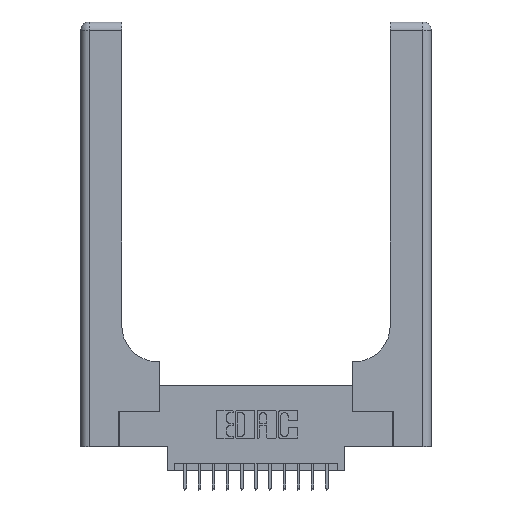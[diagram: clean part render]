
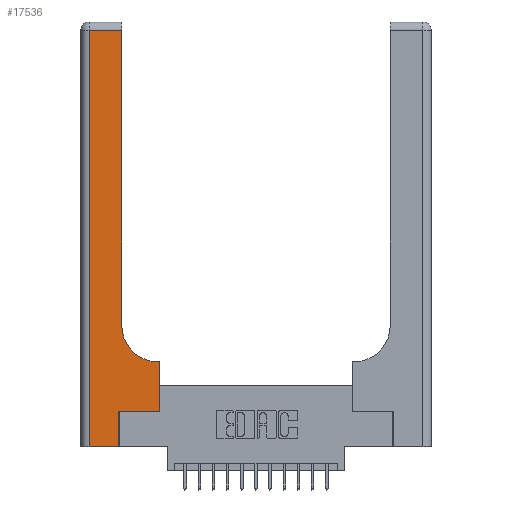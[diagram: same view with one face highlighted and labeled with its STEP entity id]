
A CAD part, top view. The second image highlights one B-rep face of the part: STEP entity #17536.
In plain terms, the highlighted planar face has unit normal (0, 0, 1).
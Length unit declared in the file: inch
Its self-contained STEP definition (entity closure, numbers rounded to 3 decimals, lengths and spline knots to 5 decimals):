
#185 = CIRCLE ( 'NONE', #14574, 0.25 ) ;
#428 = VERTEX_POINT ( 'NONE', #13243 ) ;
#440 = DIRECTION ( 'NONE',  ( 1., 0., 0. ) ) ;
#572 = LINE ( 'NONE', #4904, #17572 ) ;
#699 = EDGE_LOOP ( 'NONE', ( #13383, #5843, #14228, #2936, #4635, #8428, #7932, #6070, #11834 ) ) ;
#736 = LINE ( 'NONE', #6343, #16809 ) ;
#1186 = CARTESIAN_POINT ( 'NONE',  ( 0., 0., 0.37 ) ) ;
#1475 = EDGE_CURVE ( 'NONE', #5030, #13446, #18220, .T. ) ;
#1550 = VECTOR ( 'NONE', #15448, 39.37008 ) ;
#1582 = LINE ( 'NONE', #9690, #9158 ) ;
#1612 = DIRECTION ( 'NONE',  ( 0., -1., 0. ) ) ;
#1633 = VECTOR ( 'NONE', #12457, 39.37008 ) ;
#1812 = CARTESIAN_POINT ( 'NONE',  ( 0.5415, 0.85, 0.37 ) ) ;
#2524 = CARTESIAN_POINT ( 'NONE',  ( 0.269, 0.25, 0.37 ) ) ;
#2936 = ORIENTED_EDGE ( 'NONE', *, *, #12103, .T. ) ;
#4201 = LINE ( 'NONE', #1186, #4261 ) ;
#4261 = VECTOR ( 'NONE', #9842, 39.37008 ) ;
#4392 = VERTEX_POINT ( 'NONE', #14958 ) ;
#4635 = ORIENTED_EDGE ( 'NONE', *, *, #18204, .T. ) ;
#4637 = CARTESIAN_POINT ( 'NONE',  ( 0.269, 0., 0.37 ) ) ;
#4904 = CARTESIAN_POINT ( 'NONE',  ( 0.2915, 0.6, 0.37 ) ) ;
#5030 = VERTEX_POINT ( 'NONE', #9183 ) ;
#5843 = ORIENTED_EDGE ( 'NONE', *, *, #11168, .T. ) ;
#6070 = ORIENTED_EDGE ( 'NONE', *, *, #7329, .T. ) ;
#6343 = CARTESIAN_POINT ( 'NONE',  ( 0., 2.94, 0.37 ) ) ;
#7213 = DIRECTION ( 'NONE',  ( 0., 1., 0. ) ) ;
#7329 = EDGE_CURVE ( 'NONE', #11259, #11139, #572, .T. ) ;
#7932 = ORIENTED_EDGE ( 'NONE', *, *, #11417, .T. ) ;
#8428 = ORIENTED_EDGE ( 'NONE', *, *, #12656, .T. ) ;
#8565 = CARTESIAN_POINT ( 'NONE',  ( 0.269, 0., 0.37 ) ) ;
#9158 = VECTOR ( 'NONE', #7213, 39.37008 ) ;
#9183 = CARTESIAN_POINT ( 'NONE',  ( 0.2915, 0.85, 0.37 ) ) ;
#9417 = EDGE_CURVE ( 'NONE', #4392, #428, #15525, .T. ) ;
#9690 = CARTESIAN_POINT ( 'NONE',  ( 0.5585, 0.25, 0.37 ) ) ;
#9842 = DIRECTION ( 'NONE',  ( 1., 0., 0. ) ) ;
#10525 = VERTEX_POINT ( 'NONE', #8565 ) ;
#10575 = DIRECTION ( 'NONE',  ( -1., 0., 0. ) ) ;
#11135 = VECTOR ( 'NONE', #11459, 39.37008 ) ;
#11139 = VERTEX_POINT ( 'NONE', #12062 ) ;
#11168 = EDGE_CURVE ( 'NONE', #13446, #4392, #736, .T. ) ;
#11259 = VERTEX_POINT ( 'NONE', #16172 ) ;
#11359 = CARTESIAN_POINT ( 'NONE',  ( 0.269, 0.25, 0.37 ) ) ;
#11386 = CARTESIAN_POINT ( 'NONE',  ( 0.06, 3., 0.37 ) ) ;
#11417 = EDGE_CURVE ( 'NONE', #17155, #11259, #1582, .T. ) ;
#11459 = DIRECTION ( 'NONE',  ( 0., 1., 0. ) ) ;
#11491 = CARTESIAN_POINT ( 'NONE',  ( 0.2915, 2.94, 0.37 ) ) ;
#11541 = LINE ( 'NONE', #4637, #11135 ) ;
#11834 = ORIENTED_EDGE ( 'NONE', *, *, #13346, .T. ) ;
#12062 = CARTESIAN_POINT ( 'NONE',  ( 0.5415, 0.6, 0.37 ) ) ;
#12103 = EDGE_CURVE ( 'NONE', #428, #10525, #4201, .T. ) ;
#12457 = DIRECTION ( 'NONE',  ( 1., 0., 0. ) ) ;
#12656 = EDGE_CURVE ( 'NONE', #17316, #17155, #13838, .T. ) ;
#13243 = CARTESIAN_POINT ( 'NONE',  ( 0.06, 0., 0.37 ) ) ;
#13259 = DIRECTION ( 'NONE',  ( -1., 0., 0. ) ) ;
#13312 = VECTOR ( 'NONE', #1612, 39.37008 ) ;
#13346 = EDGE_CURVE ( 'NONE', #11139, #5030, #185, .T. ) ;
#13383 = ORIENTED_EDGE ( 'NONE', *, *, #1475, .T. ) ;
#13446 = VERTEX_POINT ( 'NONE', #11491 ) ;
#13838 = LINE ( 'NONE', #2524, #1633 ) ;
#14046 = AXIS2_PLACEMENT_3D ( 'NONE', #17228, #16009, #13259 ) ;
#14228 = ORIENTED_EDGE ( 'NONE', *, *, #9417, .T. ) ;
#14296 = CARTESIAN_POINT ( 'NONE',  ( 0.5585, 0.25, 0.37 ) ) ;
#14574 = AXIS2_PLACEMENT_3D ( 'NONE', #1812, #17297, #440 ) ;
#14958 = CARTESIAN_POINT ( 'NONE',  ( 0.06, 2.94, 0.37 ) ) ;
#15448 = DIRECTION ( 'NONE',  ( 0., 1., 0. ) ) ;
#15525 = LINE ( 'NONE', #11386, #13312 ) ;
#15918 = PLANE ( 'NONE',  #14046 ) ;
#16009 = DIRECTION ( 'NONE',  ( 0., 0., -1. ) ) ;
#16105 = FACE_OUTER_BOUND ( 'NONE', #699, .T. ) ;
#16172 = CARTESIAN_POINT ( 'NONE',  ( 0.5585, 0.6, 0.37 ) ) ;
#16229 = DIRECTION ( 'NONE',  ( -1., 0., 0. ) ) ;
#16809 = VECTOR ( 'NONE', #10575, 39.37008 ) ;
#17155 = VERTEX_POINT ( 'NONE', #14296 ) ;
#17228 = CARTESIAN_POINT ( 'NONE',  ( 0., 3., 0.37 ) ) ;
#17297 = DIRECTION ( 'NONE',  ( 0., 0., -1. ) ) ;
#17316 = VERTEX_POINT ( 'NONE', #11359 ) ;
#17536 = ADVANCED_FACE ( 'NONE', ( #16105 ), #15918, .F. ) ;
#17572 = VECTOR ( 'NONE', #16229, 39.37008 ) ;
#18123 = CARTESIAN_POINT ( 'NONE',  ( 0.2915, 3., 0.37 ) ) ;
#18204 = EDGE_CURVE ( 'NONE', #10525, #17316, #11541, .T. ) ;
#18220 = LINE ( 'NONE', #18123, #1550 ) ;
